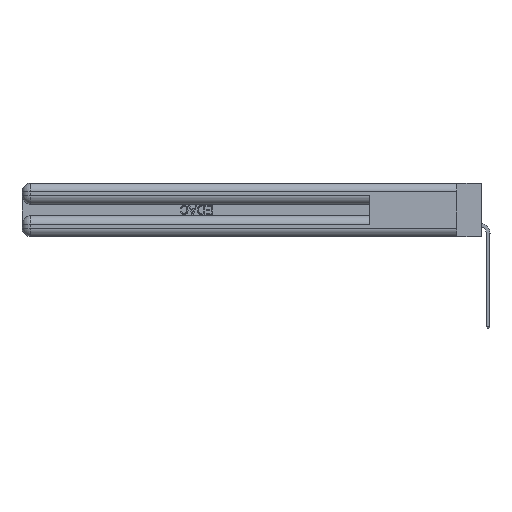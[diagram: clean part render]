
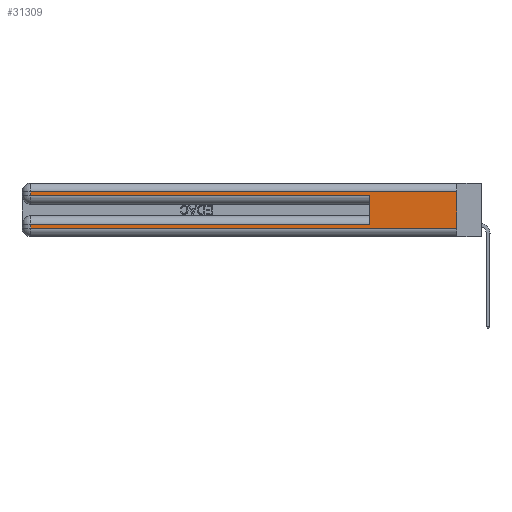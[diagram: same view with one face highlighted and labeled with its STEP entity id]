
A CAD part, left-side view. The second image highlights one B-rep face of the part: STEP entity #31309.
In plain terms, the highlighted planar face has unit normal (-1, 0, 0).
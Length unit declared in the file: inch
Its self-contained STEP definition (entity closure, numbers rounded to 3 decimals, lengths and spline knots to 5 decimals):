
#1583 = LINE ( 'NONE', #23659, #9727 ) ;
#2478 = VERTEX_POINT ( 'NONE', #16553 ) ;
#2638 = ORIENTED_EDGE ( 'NONE', *, *, #41566, .T. ) ;
#2886 = CARTESIAN_POINT ( 'NONE',  ( 0., 2.94, 0.37 ) ) ;
#3382 = VECTOR ( 'NONE', #17997, 39.37008 ) ;
#3403 = DIRECTION ( 'NONE',  ( 0., 0., -1. ) ) ;
#4624 = DIRECTION ( 'NONE',  ( 0., 1., 0. ) ) ;
#6015 = DIRECTION ( 'NONE',  ( 0., 0., -1. ) ) ;
#6452 = DIRECTION ( 'NONE',  ( 0., 1., 0. ) ) ;
#6899 = LINE ( 'NONE', #37518, #3382 ) ;
#8266 = VECTOR ( 'NONE', #22853, 39.37008 ) ;
#8273 = ORIENTED_EDGE ( 'NONE', *, *, #32655, .T. ) ;
#9727 = VECTOR ( 'NONE', #4624, 39.37008 ) ;
#10707 = VECTOR ( 'NONE', #6015, 39.37008 ) ;
#13577 = CARTESIAN_POINT ( 'NONE',  ( 0., 0., 0.06 ) ) ;
#14283 = LINE ( 'NONE', #2886, #10707 ) ;
#14474 = VECTOR ( 'NONE', #40457, 39.37008 ) ;
#16091 = VERTEX_POINT ( 'NONE', #18608 ) ;
#16553 = CARTESIAN_POINT ( 'NONE',  ( 0., 0., 0.06 ) ) ;
#17581 = PLANE ( 'NONE',  #41681 ) ;
#17997 = DIRECTION ( 'NONE',  ( 0., -1., 0. ) ) ;
#18091 = EDGE_CURVE ( 'NONE', #19617, #2478, #37113, .T. ) ;
#18448 = VECTOR ( 'NONE', #41255, 39.37008 ) ;
#18588 = EDGE_CURVE ( 'NONE', #38989, #16091, #14283, .T. ) ;
#18608 = CARTESIAN_POINT ( 'NONE',  ( 0., 2.94, 0.06 ) ) ;
#19425 = FACE_OUTER_BOUND ( 'NONE', #19659, .T. ) ;
#19437 = VERTEX_POINT ( 'NONE', #34999 ) ;
#19617 = VERTEX_POINT ( 'NONE', #28938 ) ;
#19659 = EDGE_LOOP ( 'NONE', ( #28321, #2638, #27077, #29049, #37966, #21395, #41419, #8273 ) ) ;
#19938 = LINE ( 'NONE', #26690, #14474 ) ;
#21395 = ORIENTED_EDGE ( 'NONE', *, *, #33089, .T. ) ;
#22426 = CARTESIAN_POINT ( 'NONE',  ( 0., 0., 0.31 ) ) ;
#22533 = VECTOR ( 'NONE', #6452, 39.37008 ) ;
#22853 = DIRECTION ( 'NONE',  ( 0., -1., 0. ) ) ;
#23659 = CARTESIAN_POINT ( 'NONE',  ( 0., 0., 0.085 ) ) ;
#24462 = LINE ( 'NONE', #37996, #18448 ) ;
#25441 = VECTOR ( 'NONE', #3403, 39.37008 ) ;
#26690 = CARTESIAN_POINT ( 'NONE',  ( 0., 2.94, 0.37 ) ) ;
#27067 = VERTEX_POINT ( 'NONE', #30583 ) ;
#27077 = ORIENTED_EDGE ( 'NONE', *, *, #30539, .T. ) ;
#28025 = VERTEX_POINT ( 'NONE', #35343 ) ;
#28256 = EDGE_CURVE ( 'NONE', #28025, #27067, #6899, .T. ) ;
#28321 = ORIENTED_EDGE ( 'NONE', *, *, #18091, .F. ) ;
#28938 = CARTESIAN_POINT ( 'NONE',  ( 0., 0., 0.31 ) ) ;
#29049 = ORIENTED_EDGE ( 'NONE', *, *, #28256, .T. ) ;
#29236 = CARTESIAN_POINT ( 'NONE',  ( 0., 2.94, 0.085 ) ) ;
#30539 = EDGE_CURVE ( 'NONE', #19437, #28025, #19938, .T. ) ;
#30583 = CARTESIAN_POINT ( 'NONE',  ( 0., 0.6, 0.285 ) ) ;
#31309 = ADVANCED_FACE ( 'NONE', ( #19425 ), #17581, .F. ) ;
#31495 = EDGE_CURVE ( 'NONE', #38934, #27067, #24462, .T. ) ;
#32377 = CARTESIAN_POINT ( 'NONE',  ( 0., 0., 0.37 ) ) ;
#32655 = EDGE_CURVE ( 'NONE', #16091, #2478, #33501, .T. ) ;
#33089 = EDGE_CURVE ( 'NONE', #38934, #38989, #1583, .T. ) ;
#33377 = CARTESIAN_POINT ( 'NONE',  ( 0., 0., 0.37 ) ) ;
#33501 = LINE ( 'NONE', #13577, #8266 ) ;
#34425 = CARTESIAN_POINT ( 'NONE',  ( 0., 0.6, 0.085 ) ) ;
#34999 = CARTESIAN_POINT ( 'NONE',  ( 0., 2.94, 0.31 ) ) ;
#35343 = CARTESIAN_POINT ( 'NONE',  ( 0., 2.94, 0.285 ) ) ;
#35699 = LINE ( 'NONE', #22426, #22533 ) ;
#36975 = DIRECTION ( 'NONE',  ( 1., 0., 0. ) ) ;
#37113 = LINE ( 'NONE', #32377, #25441 ) ;
#37518 = CARTESIAN_POINT ( 'NONE',  ( 0., 0., 0.285 ) ) ;
#37966 = ORIENTED_EDGE ( 'NONE', *, *, #31495, .F. ) ;
#37996 = CARTESIAN_POINT ( 'NONE',  ( 0., 0.6, 0.145 ) ) ;
#38934 = VERTEX_POINT ( 'NONE', #34425 ) ;
#38989 = VERTEX_POINT ( 'NONE', #29236 ) ;
#40457 = DIRECTION ( 'NONE',  ( 0., 0., -1. ) ) ;
#40527 = DIRECTION ( 'NONE',  ( 0., 0., -1. ) ) ;
#41255 = DIRECTION ( 'NONE',  ( 0., 0., 1. ) ) ;
#41419 = ORIENTED_EDGE ( 'NONE', *, *, #18588, .T. ) ;
#41566 = EDGE_CURVE ( 'NONE', #19617, #19437, #35699, .T. ) ;
#41681 = AXIS2_PLACEMENT_3D ( 'NONE', #33377, #36975, #40527 ) ;
